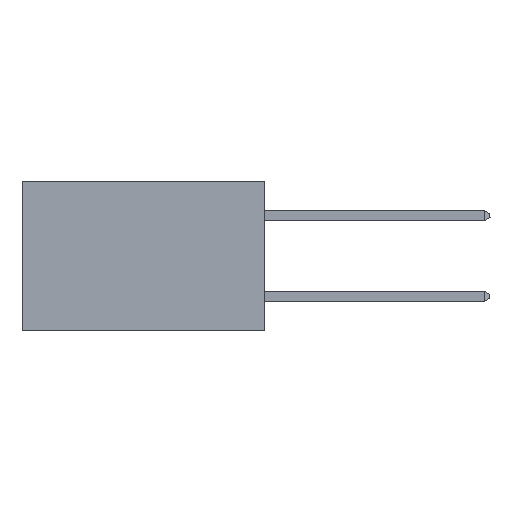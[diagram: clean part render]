
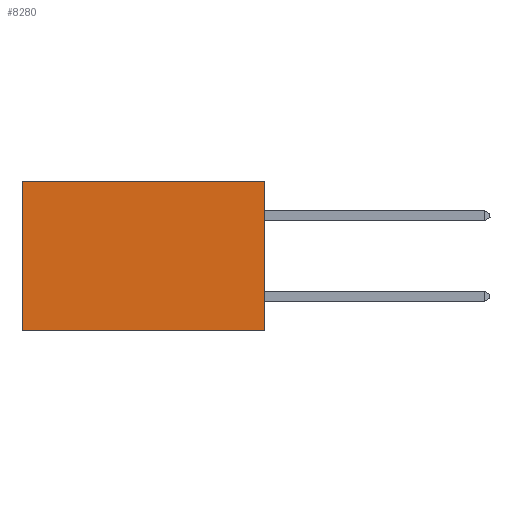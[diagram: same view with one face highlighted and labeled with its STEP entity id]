
A CAD part, left-side view. The second image highlights one B-rep face of the part: STEP entity #8280.
In plain terms, the highlighted planar face has unit normal (-1, 0, 0).
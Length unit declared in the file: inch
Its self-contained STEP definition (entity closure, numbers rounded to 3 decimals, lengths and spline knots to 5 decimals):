
#290 = EDGE_CURVE ( 'NONE', #3160, #8206, #4493, .T. ) ;
#370 = CARTESIAN_POINT ( 'NONE',  ( 0.298, 0.6, 0. ) ) ;
#1199 = CARTESIAN_POINT ( 'NONE',  ( 0.298, 0., 0. ) ) ;
#1300 = AXIS2_PLACEMENT_3D ( 'NONE', #3830, #8759, #4566 ) ;
#1373 = FACE_OUTER_BOUND ( 'NONE', #1795, .T. ) ;
#1382 = EDGE_CURVE ( 'NONE', #4375, #5901, #2056, .T. ) ;
#1795 = EDGE_LOOP ( 'NONE', ( #5277, #1812, #7516, #5984 ) ) ;
#1812 = ORIENTED_EDGE ( 'NONE', *, *, #3700, .F. ) ;
#2056 = LINE ( 'NONE', #370, #4787 ) ;
#2229 = CARTESIAN_POINT ( 'NONE',  ( 0.298, 0.6, -0.37 ) ) ;
#2441 = LINE ( 'NONE', #6755, #5851 ) ;
#3100 = CARTESIAN_POINT ( 'NONE',  ( 0.298, 0.6, 0. ) ) ;
#3160 = VERTEX_POINT ( 'NONE', #5809 ) ;
#3700 = EDGE_CURVE ( 'NONE', #8206, #5901, #2441, .T. ) ;
#3830 = CARTESIAN_POINT ( 'NONE',  ( 0.298, 0., 0. ) ) ;
#3907 = DIRECTION ( 'NONE',  ( 0., 1., 0. ) ) ;
#3995 = DIRECTION ( 'NONE',  ( 0., 0., -1. ) ) ;
#4006 = LINE ( 'NONE', #4473, #4557 ) ;
#4375 = VERTEX_POINT ( 'NONE', #3100 ) ;
#4473 = CARTESIAN_POINT ( 'NONE',  ( 0.298, 0., 0. ) ) ;
#4493 = LINE ( 'NONE', #1199, #7678 ) ;
#4557 = VECTOR ( 'NONE', #7337, 39.37008 ) ;
#4566 = DIRECTION ( 'NONE',  ( 0., 0., -1. ) ) ;
#4787 = VECTOR ( 'NONE', #6672, 39.37008 ) ;
#5277 = ORIENTED_EDGE ( 'NONE', *, *, #1382, .T. ) ;
#5809 = CARTESIAN_POINT ( 'NONE',  ( 0.298, 0., 0. ) ) ;
#5851 = VECTOR ( 'NONE', #3907, 39.37008 ) ;
#5901 = VERTEX_POINT ( 'NONE', #2229 ) ;
#5984 = ORIENTED_EDGE ( 'NONE', *, *, #7224, .T. ) ;
#6672 = DIRECTION ( 'NONE',  ( 0., 0., -1. ) ) ;
#6755 = CARTESIAN_POINT ( 'NONE',  ( 0.298, 0., -0.37 ) ) ;
#7224 = EDGE_CURVE ( 'NONE', #3160, #4375, #4006, .T. ) ;
#7337 = DIRECTION ( 'NONE',  ( 0., 1., 0. ) ) ;
#7516 = ORIENTED_EDGE ( 'NONE', *, *, #290, .F. ) ;
#7678 = VECTOR ( 'NONE', #3995, 39.37008 ) ;
#8135 = CARTESIAN_POINT ( 'NONE',  ( 0.298, 0., -0.37 ) ) ;
#8206 = VERTEX_POINT ( 'NONE', #8135 ) ;
#8280 = ADVANCED_FACE ( 'NONE', ( #1373 ), #8837, .F. ) ;
#8759 = DIRECTION ( 'NONE',  ( 1., 0., 0. ) ) ;
#8837 = PLANE ( 'NONE',  #1300 ) ;
